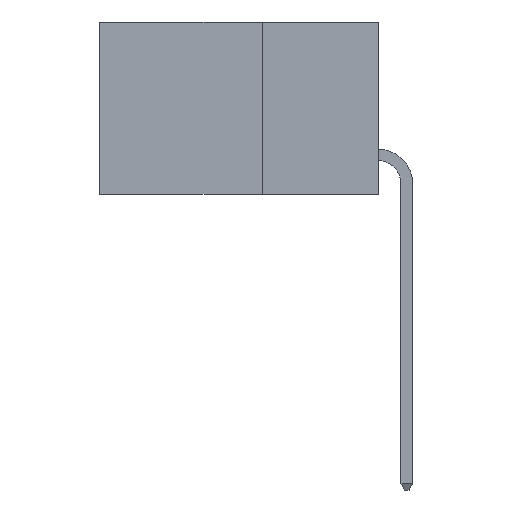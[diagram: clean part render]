
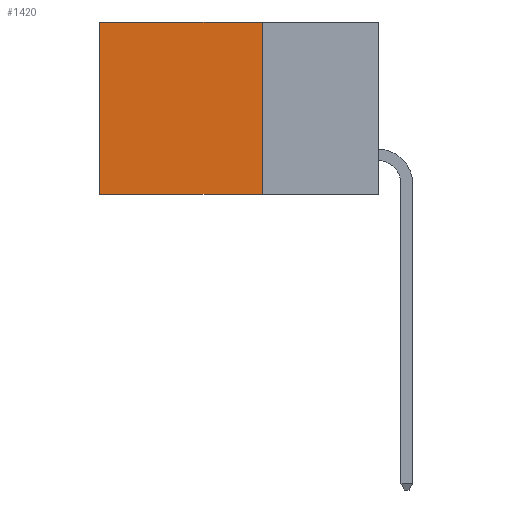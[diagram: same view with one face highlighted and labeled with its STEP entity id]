
A CAD part, left-side view. The second image highlights one B-rep face of the part: STEP entity #1420.
In plain terms, the highlighted planar face has unit normal (-1, 0, 0).
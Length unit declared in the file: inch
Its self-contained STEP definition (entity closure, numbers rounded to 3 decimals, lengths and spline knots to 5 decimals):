
#478 = DIRECTION ( 'NONE',  ( 0., 0., -1. ) ) ;
#952 = PLANE ( 'NONE',  #9744 ) ;
#1003 = CARTESIAN_POINT ( 'NONE',  ( 0.2615, 0.25, -0.37 ) ) ;
#1202 = EDGE_CURVE ( 'NONE', #9693, #1342, #1769, .T. ) ;
#1250 = CARTESIAN_POINT ( 'NONE',  ( 0.2615, 0.25, -0.37 ) ) ;
#1342 = VERTEX_POINT ( 'NONE', #6447 ) ;
#1420 = ADVANCED_FACE ( 'NONE', ( #2074 ), #952, .F. ) ;
#1510 = CARTESIAN_POINT ( 'NONE',  ( 0.2615, 0.25, -0.37 ) ) ;
#1529 = ORIENTED_EDGE ( 'NONE', *, *, #9486, .T. ) ;
#1769 = LINE ( 'NONE', #2325, #10078 ) ;
#1854 = VERTEX_POINT ( 'NONE', #4350 ) ;
#2074 = FACE_OUTER_BOUND ( 'NONE', #9420, .T. ) ;
#2080 = DIRECTION ( 'NONE',  ( 0., 1., 0. ) ) ;
#2325 = CARTESIAN_POINT ( 'NONE',  ( 0.2615, 0.25, -0.37 ) ) ;
#2462 = DIRECTION ( 'NONE',  ( 0., 0., -1. ) ) ;
#2463 = VECTOR ( 'NONE', #9889, 39.37008 ) ;
#3131 = VECTOR ( 'NONE', #2080, 39.37008 ) ;
#4019 = EDGE_CURVE ( 'NONE', #1854, #9693, #4828, .T. ) ;
#4024 = EDGE_CURVE ( 'NONE', #1854, #5997, #6992, .T. ) ;
#4082 = ORIENTED_EDGE ( 'NONE', *, *, #1202, .F. ) ;
#4350 = CARTESIAN_POINT ( 'NONE',  ( 0.2615, 0.25, 0. ) ) ;
#4374 = VECTOR ( 'NONE', #478, 39.37008 ) ;
#4818 = DIRECTION ( 'NONE',  ( 1., 0., 0. ) ) ;
#4828 = LINE ( 'NONE', #1510, #2463 ) ;
#5997 = VERTEX_POINT ( 'NONE', #10819 ) ;
#6279 = ORIENTED_EDGE ( 'NONE', *, *, #4019, .F. ) ;
#6447 = CARTESIAN_POINT ( 'NONE',  ( 0.2615, 0.6, -0.37 ) ) ;
#6615 = DIRECTION ( 'NONE',  ( 0., 1., 0. ) ) ;
#6992 = LINE ( 'NONE', #9873, #3131 ) ;
#9420 = EDGE_LOOP ( 'NONE', ( #1529, #4082, #6279, #10351 ) ) ;
#9486 = EDGE_CURVE ( 'NONE', #5997, #1342, #10604, .T. ) ;
#9620 = CARTESIAN_POINT ( 'NONE',  ( 0.2615, 0.6, -0.37 ) ) ;
#9693 = VERTEX_POINT ( 'NONE', #1250 ) ;
#9744 = AXIS2_PLACEMENT_3D ( 'NONE', #1003, #4818, #2462 ) ;
#9873 = CARTESIAN_POINT ( 'NONE',  ( 0.2615, 0.25, 0. ) ) ;
#9889 = DIRECTION ( 'NONE',  ( 0., 0., -1. ) ) ;
#10078 = VECTOR ( 'NONE', #6615, 39.37008 ) ;
#10351 = ORIENTED_EDGE ( 'NONE', *, *, #4024, .T. ) ;
#10604 = LINE ( 'NONE', #9620, #4374 ) ;
#10819 = CARTESIAN_POINT ( 'NONE',  ( 0.2615, 0.6, 0. ) ) ;
